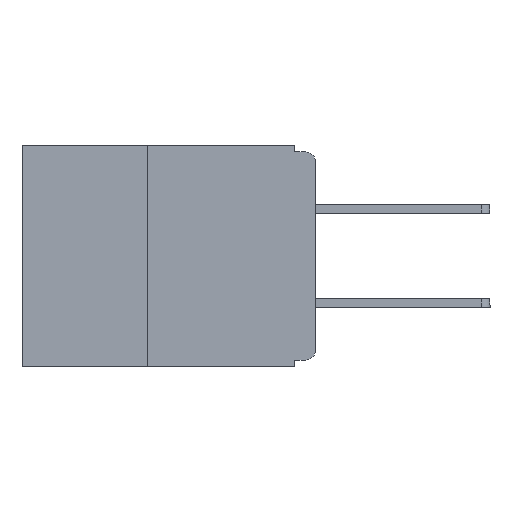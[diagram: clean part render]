
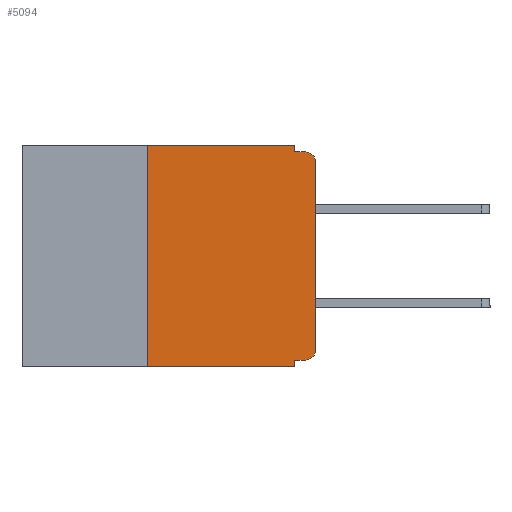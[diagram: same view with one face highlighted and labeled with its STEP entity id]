
A CAD part, left-side view. The second image highlights one B-rep face of the part: STEP entity #5094.
In plain terms, the highlighted planar face has unit normal (-1, 0, 0).
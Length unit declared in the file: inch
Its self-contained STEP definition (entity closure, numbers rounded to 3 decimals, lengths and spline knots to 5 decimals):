
#190 = LINE ( 'NONE', #9518, #15365 ) ;
#424 = LINE ( 'NONE', #17589, #14979 ) ;
#613 = VERTEX_POINT ( 'NONE', #11626 ) ;
#663 = DIRECTION ( 'NONE',  ( 0., 0., -1. ) ) ;
#835 = EDGE_CURVE ( 'NONE', #24581, #1490, #25410, .T. ) ;
#1283 = DIRECTION ( 'NONE',  ( 0., 0., -1. ) ) ;
#1490 = VERTEX_POINT ( 'NONE', #15749 ) ;
#2007 = VERTEX_POINT ( 'NONE', #2791 ) ;
#2051 = EDGE_CURVE ( 'NONE', #24004, #2007, #9261, .T. ) ;
#2337 = CARTESIAN_POINT ( 'NONE',  ( 0., 0.031, 0. ) ) ;
#2427 = DIRECTION ( 'NONE',  ( 0., -1., 0. ) ) ;
#2477 = CARTESIAN_POINT ( 'NONE',  ( 0., 0.031, -0.32 ) ) ;
#2791 = CARTESIAN_POINT ( 'NONE',  ( 0., 0.031, -0.33 ) ) ;
#3139 = LINE ( 'NONE', #20793, #23965 ) ;
#3202 = FACE_OUTER_BOUND ( 'NONE', #7165, .T. ) ;
#3294 = VERTEX_POINT ( 'NONE', #4750 ) ;
#4455 = LINE ( 'NONE', #18365, #14321 ) ;
#4644 = VECTOR ( 'NONE', #663, 39.37008 ) ;
#4667 = LINE ( 'NONE', #22554, #24815 ) ;
#4750 = CARTESIAN_POINT ( 'NONE',  ( 0., 0.25, -0.33 ) ) ;
#4797 = VECTOR ( 'NONE', #2427, 39.37008 ) ;
#5028 = EDGE_CURVE ( 'NONE', #3294, #2007, #4455, .T. ) ;
#5094 = ADVANCED_FACE ( 'NONE', ( #3202 ), #17686, .F. ) ;
#5274 = VECTOR ( 'NONE', #20568, 39.37008 ) ;
#5430 = LINE ( 'NONE', #18202, #4797 ) ;
#5575 = VERTEX_POINT ( 'NONE', #11243 ) ;
#5583 = CIRCLE ( 'NONE', #23690, 0.015 ) ;
#5704 = CARTESIAN_POINT ( 'NONE',  ( 0., 0., -0.025 ) ) ;
#6557 = EDGE_CURVE ( 'NONE', #613, #24004, #4667, .T. ) ;
#6700 = CARTESIAN_POINT ( 'NONE',  ( 0., 0.031, -0.01 ) ) ;
#6853 = VERTEX_POINT ( 'NONE', #13150 ) ;
#7165 = EDGE_LOOP ( 'NONE', ( #14066, #15653, #16074, #16219, #16719, #16779, #17073, #19702, #20982, #21355 ) ) ;
#9261 = LINE ( 'NONE', #13405, #4644 ) ;
#9518 = CARTESIAN_POINT ( 'NONE',  ( 0., 0., 0. ) ) ;
#10715 = DIRECTION ( 'NONE',  ( -1., 0., 0. ) ) ;
#11243 = CARTESIAN_POINT ( 'NONE',  ( 0., 0.25, 0. ) ) ;
#11444 = VERTEX_POINT ( 'NONE', #2337 ) ;
#11626 = CARTESIAN_POINT ( 'NONE',  ( 0., 0.015, -0.32 ) ) ;
#11916 = EDGE_CURVE ( 'NONE', #3294, #5575, #424, .T. ) ;
#12821 = EDGE_CURVE ( 'NONE', #5575, #11444, #5430, .T. ) ;
#13131 = DIRECTION ( 'NONE',  ( -1., 0., 0. ) ) ;
#13150 = CARTESIAN_POINT ( 'NONE',  ( 0., 0., -0.305 ) ) ;
#13405 = CARTESIAN_POINT ( 'NONE',  ( 0., 0.031, -0.33 ) ) ;
#14066 = ORIENTED_EDGE ( 'NONE', *, *, #18767, .T. ) ;
#14321 = VECTOR ( 'NONE', #18289, 39.37008 ) ;
#14883 = EDGE_CURVE ( 'NONE', #11444, #24581, #3139, .T. ) ;
#14979 = VECTOR ( 'NONE', #19520, 39.37008 ) ;
#15012 = DIRECTION ( 'NONE',  ( 0., 0., -1. ) ) ;
#15365 = VECTOR ( 'NONE', #23174, 39.37008 ) ;
#15653 = ORIENTED_EDGE ( 'NONE', *, *, #15681, .T. ) ;
#15681 = EDGE_CURVE ( 'NONE', #19475, #1490, #5583, .T. ) ;
#15749 = CARTESIAN_POINT ( 'NONE',  ( 0., 0.015, -0.01 ) ) ;
#16074 = ORIENTED_EDGE ( 'NONE', *, *, #835, .F. ) ;
#16219 = ORIENTED_EDGE ( 'NONE', *, *, #14883, .F. ) ;
#16719 = ORIENTED_EDGE ( 'NONE', *, *, #12821, .F. ) ;
#16779 = ORIENTED_EDGE ( 'NONE', *, *, #11916, .F. ) ;
#16863 = AXIS2_PLACEMENT_3D ( 'NONE', #18128, #17627, #17602 ) ;
#17073 = ORIENTED_EDGE ( 'NONE', *, *, #5028, .T. ) ;
#17268 = AXIS2_PLACEMENT_3D ( 'NONE', #24762, #13131, #1283 ) ;
#17589 = CARTESIAN_POINT ( 'NONE',  ( 0., 0.25, -0.33 ) ) ;
#17602 = DIRECTION ( 'NONE',  ( 0., 0., -1. ) ) ;
#17627 = DIRECTION ( 'NONE',  ( 1., 0., 0. ) ) ;
#17686 = PLANE ( 'NONE',  #16863 ) ;
#18128 = CARTESIAN_POINT ( 'NONE',  ( 0., 0.437, 0. ) ) ;
#18202 = CARTESIAN_POINT ( 'NONE',  ( 0., 0.437, 0. ) ) ;
#18289 = DIRECTION ( 'NONE',  ( 0., -1., 0. ) ) ;
#18365 = CARTESIAN_POINT ( 'NONE',  ( 0., 0.437, -0.33 ) ) ;
#18767 = EDGE_CURVE ( 'NONE', #6853, #19475, #190, .T. ) ;
#19475 = VERTEX_POINT ( 'NONE', #5704 ) ;
#19520 = DIRECTION ( 'NONE',  ( 0., 0., 1. ) ) ;
#19702 = ORIENTED_EDGE ( 'NONE', *, *, #2051, .F. ) ;
#20006 = CARTESIAN_POINT ( 'NONE',  ( 0., 0., -0.01 ) ) ;
#20568 = DIRECTION ( 'NONE',  ( 0., -1., 0. ) ) ;
#20793 = CARTESIAN_POINT ( 'NONE',  ( 0., 0.031, 0. ) ) ;
#20982 = ORIENTED_EDGE ( 'NONE', *, *, #6557, .F. ) ;
#21355 = ORIENTED_EDGE ( 'NONE', *, *, #23357, .T. ) ;
#21982 = DIRECTION ( 'NONE',  ( 0., 1., 0. ) ) ;
#22441 = CARTESIAN_POINT ( 'NONE',  ( 0., 0.015, -0.025 ) ) ;
#22554 = CARTESIAN_POINT ( 'NONE',  ( 0., 0., -0.32 ) ) ;
#23174 = DIRECTION ( 'NONE',  ( 0., 0., 1. ) ) ;
#23357 = EDGE_CURVE ( 'NONE', #613, #6853, #24223, .T. ) ;
#23690 = AXIS2_PLACEMENT_3D ( 'NONE', #22441, #10715, #24323 ) ;
#23965 = VECTOR ( 'NONE', #15012, 39.37008 ) ;
#24004 = VERTEX_POINT ( 'NONE', #2477 ) ;
#24223 = CIRCLE ( 'NONE', #17268, 0.015 ) ;
#24323 = DIRECTION ( 'NONE',  ( 0., 0., -1. ) ) ;
#24581 = VERTEX_POINT ( 'NONE', #6700 ) ;
#24762 = CARTESIAN_POINT ( 'NONE',  ( 0., 0.015, -0.305 ) ) ;
#24815 = VECTOR ( 'NONE', #21982, 39.37008 ) ;
#25410 = LINE ( 'NONE', #20006, #5274 ) ;
